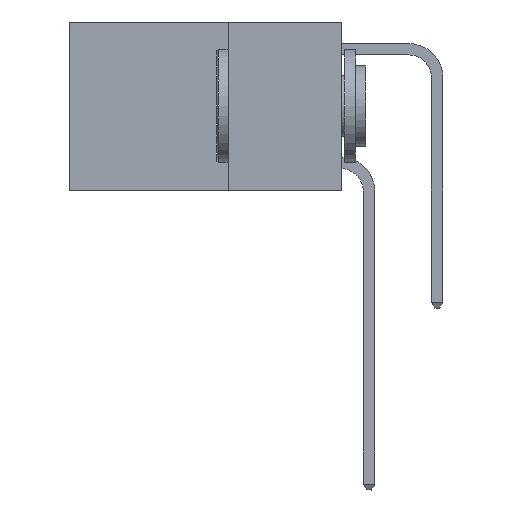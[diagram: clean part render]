
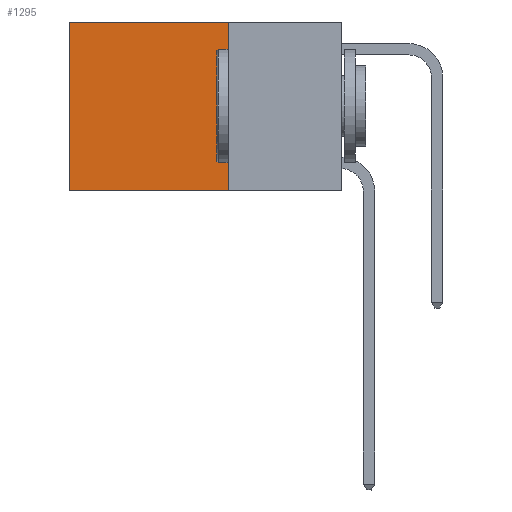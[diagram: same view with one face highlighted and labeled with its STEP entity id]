
A CAD part, left-side view. The second image highlights one B-rep face of the part: STEP entity #1295.
In plain terms, the highlighted planar face has unit normal (-1, 0, 0).
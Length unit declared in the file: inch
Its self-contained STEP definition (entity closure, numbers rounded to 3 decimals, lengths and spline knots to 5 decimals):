
#387 = ORIENTED_EDGE ( 'NONE', *, *, #6790, .T. ) ;
#656 = CARTESIAN_POINT ( 'NONE',  ( 0.2625, 0.25, 0. ) ) ;
#1295 = ADVANCED_FACE ( 'NONE', ( #2586 ), #16183, .F. ) ;
#1472 = LINE ( 'NONE', #11310, #2696 ) ;
#2174 = EDGE_LOOP ( 'NONE', ( #387, #6988, #16819, #8451 ) ) ;
#2586 = FACE_OUTER_BOUND ( 'NONE', #2174, .T. ) ;
#2696 = VECTOR ( 'NONE', #3229, 39.37008 ) ;
#3229 = DIRECTION ( 'NONE',  ( 0., 1., 0. ) ) ;
#4228 = VERTEX_POINT ( 'NONE', #19782 ) ;
#5365 = EDGE_CURVE ( 'NONE', #16740, #11152, #1472, .T. ) ;
#6612 = EDGE_CURVE ( 'NONE', #17457, #16740, #18607, .T. ) ;
#6790 = EDGE_CURVE ( 'NONE', #4228, #11152, #14433, .T. ) ;
#6988 = ORIENTED_EDGE ( 'NONE', *, *, #5365, .F. ) ;
#8145 = CARTESIAN_POINT ( 'NONE',  ( 0.2625, 0.25, 0. ) ) ;
#8451 = ORIENTED_EDGE ( 'NONE', *, *, #17796, .T. ) ;
#8589 = CARTESIAN_POINT ( 'NONE',  ( 0.2625, 0.25, 0. ) ) ;
#10064 = DIRECTION ( 'NONE',  ( 0., 1., 0. ) ) ;
#10158 = VECTOR ( 'NONE', #11827, 39.37008 ) ;
#10501 = CARTESIAN_POINT ( 'NONE',  ( 0.2625, 0.25, -0.37 ) ) ;
#10717 = LINE ( 'NONE', #8589, #15213 ) ;
#10868 = CARTESIAN_POINT ( 'NONE',  ( 0.2625, 0.25, 0. ) ) ;
#11152 = VERTEX_POINT ( 'NONE', #16392 ) ;
#11310 = CARTESIAN_POINT ( 'NONE',  ( 0.2625, 0.25, -0.37 ) ) ;
#11429 = DIRECTION ( 'NONE',  ( 1., 0., 0. ) ) ;
#11827 = DIRECTION ( 'NONE',  ( 0., 0., -1. ) ) ;
#13790 = DIRECTION ( 'NONE',  ( 0., 0., -1. ) ) ;
#14433 = LINE ( 'NONE', #19880, #18850 ) ;
#15213 = VECTOR ( 'NONE', #10064, 39.37008 ) ;
#16183 = PLANE ( 'NONE',  #17075 ) ;
#16392 = CARTESIAN_POINT ( 'NONE',  ( 0.2625, 0.6, -0.37 ) ) ;
#16740 = VERTEX_POINT ( 'NONE', #10501 ) ;
#16819 = ORIENTED_EDGE ( 'NONE', *, *, #6612, .F. ) ;
#17075 = AXIS2_PLACEMENT_3D ( 'NONE', #8145, #11429, #17701 ) ;
#17457 = VERTEX_POINT ( 'NONE', #10868 ) ;
#17701 = DIRECTION ( 'NONE',  ( 0., 0., -1. ) ) ;
#17796 = EDGE_CURVE ( 'NONE', #17457, #4228, #10717, .T. ) ;
#18607 = LINE ( 'NONE', #656, #10158 ) ;
#18850 = VECTOR ( 'NONE', #13790, 39.37008 ) ;
#19782 = CARTESIAN_POINT ( 'NONE',  ( 0.2625, 0.6, 0. ) ) ;
#19880 = CARTESIAN_POINT ( 'NONE',  ( 0.2625, 0.6, 0. ) ) ;
